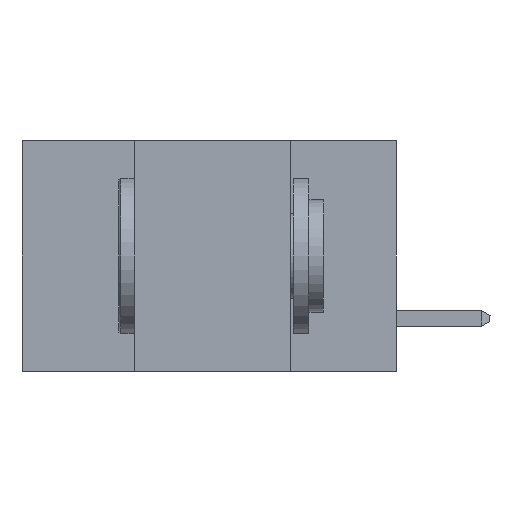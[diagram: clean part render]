
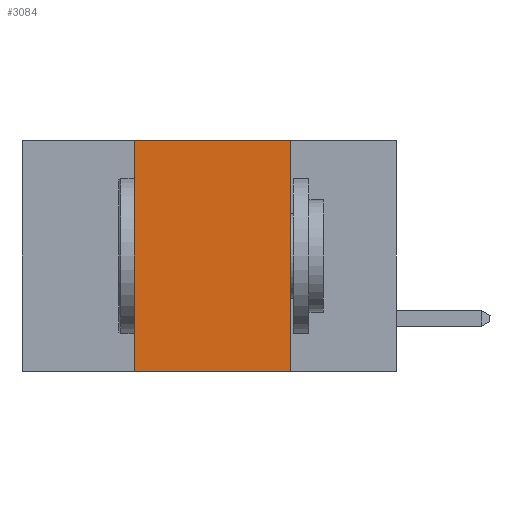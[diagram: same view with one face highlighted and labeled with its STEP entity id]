
A CAD part, left-side view. The second image highlights one B-rep face of the part: STEP entity #3084.
In plain terms, the highlighted planar face has unit normal (-1, 0, 0).
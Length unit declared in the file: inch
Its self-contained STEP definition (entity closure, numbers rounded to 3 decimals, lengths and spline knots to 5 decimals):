
#567 = LINE ( 'NONE', #7233, #18415 ) ;
#931 = VERTEX_POINT ( 'NONE', #20021 ) ;
#1934 = CARTESIAN_POINT ( 'NONE',  ( 0., 0.17, 0. ) ) ;
#2025 = DIRECTION ( 'NONE',  ( 0., 0., -1. ) ) ;
#2909 = VECTOR ( 'NONE', #2025, 39.37008 ) ;
#3084 = ADVANCED_FACE ( 'NONE', ( #19182 ), #4134, .F. ) ;
#3461 = DIRECTION ( 'NONE',  ( 0., 0., -1. ) ) ;
#3561 = DIRECTION ( 'NONE',  ( 1., 0., 0. ) ) ;
#3619 = CARTESIAN_POINT ( 'NONE',  ( 0., 0.6, 0. ) ) ;
#4004 = EDGE_LOOP ( 'NONE', ( #20273, #11358, #19766, #5594 ) ) ;
#4134 = PLANE ( 'NONE',  #6303 ) ;
#4740 = VECTOR ( 'NONE', #19034, 39.37008 ) ;
#5594 = ORIENTED_EDGE ( 'NONE', *, *, #20861, .T. ) ;
#6303 = AXIS2_PLACEMENT_3D ( 'NONE', #3619, #3561, #3461 ) ;
#6485 = LINE ( 'NONE', #15212, #19571 ) ;
#7233 = CARTESIAN_POINT ( 'NONE',  ( 0., 0.6, 0. ) ) ;
#7255 = DIRECTION ( 'NONE',  ( 0., -1., 0. ) ) ;
#9466 = LINE ( 'NONE', #17733, #4740 ) ;
#9891 = EDGE_CURVE ( 'NONE', #17922, #11581, #567, .T. ) ;
#10318 = EDGE_CURVE ( 'NONE', #13432, #17922, #9466, .T. ) ;
#11358 = ORIENTED_EDGE ( 'NONE', *, *, #9891, .F. ) ;
#11581 = VERTEX_POINT ( 'NONE', #1934 ) ;
#13432 = VERTEX_POINT ( 'NONE', #21514 ) ;
#14495 = EDGE_CURVE ( 'NONE', #11581, #931, #21124, .T. ) ;
#15212 = CARTESIAN_POINT ( 'NONE',  ( 0., 0.6, -0.37 ) ) ;
#16907 = DIRECTION ( 'NONE',  ( 0., -1., 0. ) ) ;
#17733 = CARTESIAN_POINT ( 'NONE',  ( 0., 0.42, -0.37 ) ) ;
#17922 = VERTEX_POINT ( 'NONE', #19279 ) ;
#18415 = VECTOR ( 'NONE', #7255, 39.37008 ) ;
#19034 = DIRECTION ( 'NONE',  ( 0., 0., 1. ) ) ;
#19182 = FACE_OUTER_BOUND ( 'NONE', #4004, .T. ) ;
#19279 = CARTESIAN_POINT ( 'NONE',  ( 0., 0.42, 0. ) ) ;
#19571 = VECTOR ( 'NONE', #16907, 39.37008 ) ;
#19766 = ORIENTED_EDGE ( 'NONE', *, *, #10318, .F. ) ;
#20021 = CARTESIAN_POINT ( 'NONE',  ( 0., 0.17, -0.37 ) ) ;
#20273 = ORIENTED_EDGE ( 'NONE', *, *, #14495, .F. ) ;
#20861 = EDGE_CURVE ( 'NONE', #13432, #931, #6485, .T. ) ;
#20916 = CARTESIAN_POINT ( 'NONE',  ( 0., 0.17, -0.37 ) ) ;
#21124 = LINE ( 'NONE', #20916, #2909 ) ;
#21514 = CARTESIAN_POINT ( 'NONE',  ( 0., 0.42, -0.37 ) ) ;
